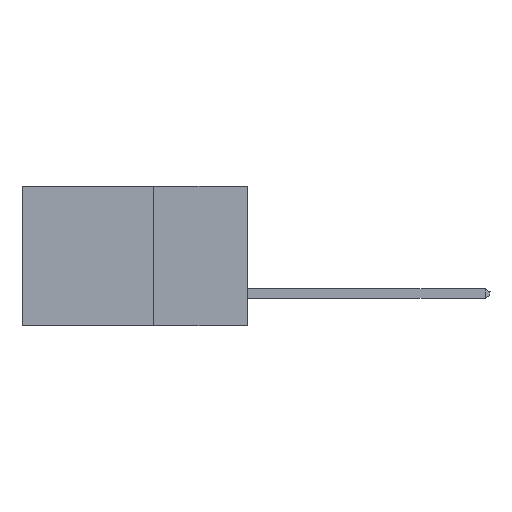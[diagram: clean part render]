
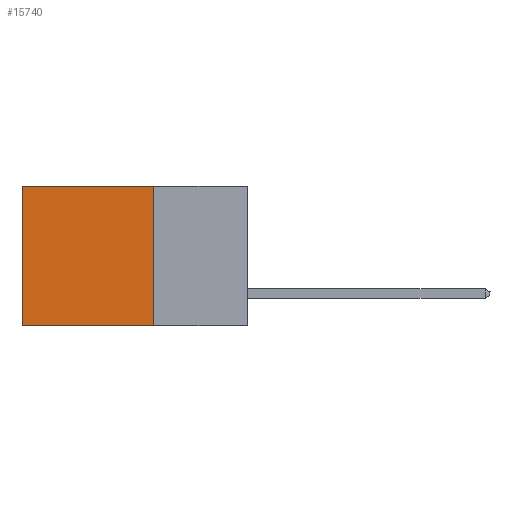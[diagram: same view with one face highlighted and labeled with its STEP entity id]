
A CAD part, left-side view. The second image highlights one B-rep face of the part: STEP entity #15740.
In plain terms, the highlighted planar face has unit normal (-1, 0, 0).
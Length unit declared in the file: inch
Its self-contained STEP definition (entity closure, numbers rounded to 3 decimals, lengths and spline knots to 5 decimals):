
#602 = VERTEX_POINT ( 'NONE', #8280 ) ;
#1315 = EDGE_CURVE ( 'NONE', #602, #7386, #12103, .T. ) ;
#2070 = CARTESIAN_POINT ( 'NONE',  ( 0.298, 0.25, -0.37 ) ) ;
#2080 = CARTESIAN_POINT ( 'NONE',  ( 0.298, 0.6, 0. ) ) ;
#2158 = ORIENTED_EDGE ( 'NONE', *, *, #10160, .T. ) ;
#2235 = FACE_OUTER_BOUND ( 'NONE', #13211, .T. ) ;
#2548 = DIRECTION ( 'NONE',  ( 1., 0., 0. ) ) ;
#2956 = LINE ( 'NONE', #16922, #4865 ) ;
#3858 = ORIENTED_EDGE ( 'NONE', *, *, #7893, .T. ) ;
#4450 = VERTEX_POINT ( 'NONE', #17091 ) ;
#4646 = VECTOR ( 'NONE', #15374, 39.37008 ) ;
#4850 = LINE ( 'NONE', #7389, #4646 ) ;
#4865 = VECTOR ( 'NONE', #12664, 39.37008 ) ;
#4991 = CARTESIAN_POINT ( 'NONE',  ( 0.298, 0.25, 0. ) ) ;
#6045 = CARTESIAN_POINT ( 'NONE',  ( 0.298, 0.6, -0.37 ) ) ;
#7325 = VERTEX_POINT ( 'NONE', #9131 ) ;
#7386 = VERTEX_POINT ( 'NONE', #6045 ) ;
#7389 = CARTESIAN_POINT ( 'NONE',  ( 0.298, 0.25, 0. ) ) ;
#7893 = EDGE_CURVE ( 'NONE', #7325, #7386, #12183, .T. ) ;
#8280 = CARTESIAN_POINT ( 'NONE',  ( 0.298, 0.25, -0.37 ) ) ;
#8939 = DIRECTION ( 'NONE',  ( 0., 1., 0. ) ) ;
#9002 = ORIENTED_EDGE ( 'NONE', *, *, #1315, .F. ) ;
#9077 = DIRECTION ( 'NONE',  ( 0., 0., -1. ) ) ;
#9131 = CARTESIAN_POINT ( 'NONE',  ( 0.298, 0.6, 0. ) ) ;
#9880 = EDGE_CURVE ( 'NONE', #4450, #602, #2956, .T. ) ;
#10160 = EDGE_CURVE ( 'NONE', #4450, #7325, #4850, .T. ) ;
#10470 = VECTOR ( 'NONE', #9077, 39.37008 ) ;
#12103 = LINE ( 'NONE', #2070, #12312 ) ;
#12114 = DIRECTION ( 'NONE',  ( 0., 0., -1. ) ) ;
#12183 = LINE ( 'NONE', #2080, #10470 ) ;
#12312 = VECTOR ( 'NONE', #8939, 39.37008 ) ;
#12664 = DIRECTION ( 'NONE',  ( 0., 0., -1. ) ) ;
#13211 = EDGE_LOOP ( 'NONE', ( #3858, #9002, #13313, #2158 ) ) ;
#13313 = ORIENTED_EDGE ( 'NONE', *, *, #9880, .F. ) ;
#14480 = PLANE ( 'NONE',  #14945 ) ;
#14945 = AXIS2_PLACEMENT_3D ( 'NONE', #4991, #2548, #12114 ) ;
#15374 = DIRECTION ( 'NONE',  ( 0., 1., 0. ) ) ;
#15740 = ADVANCED_FACE ( 'NONE', ( #2235 ), #14480, .F. ) ;
#16922 = CARTESIAN_POINT ( 'NONE',  ( 0.298, 0.25, 0. ) ) ;
#17091 = CARTESIAN_POINT ( 'NONE',  ( 0.298, 0.25, 0. ) ) ;
